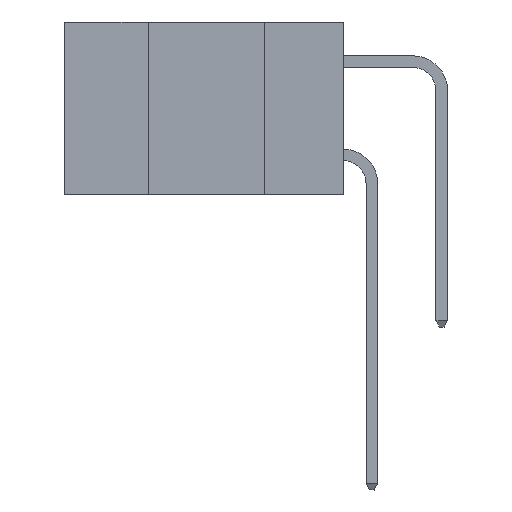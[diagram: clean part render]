
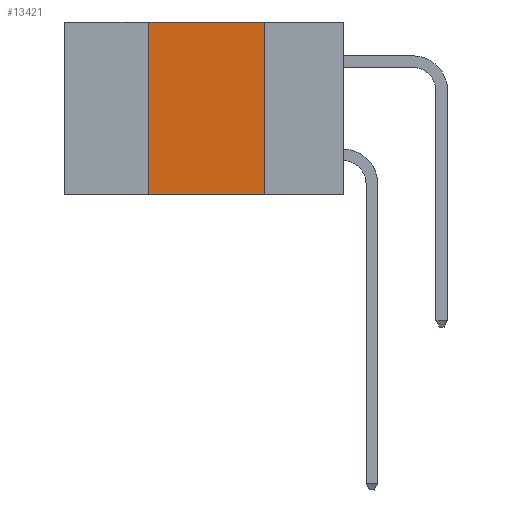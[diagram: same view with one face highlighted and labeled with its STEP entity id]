
A CAD part, left-side view. The second image highlights one B-rep face of the part: STEP entity #13421.
In plain terms, the highlighted planar face has unit normal (-1, 0, 0).
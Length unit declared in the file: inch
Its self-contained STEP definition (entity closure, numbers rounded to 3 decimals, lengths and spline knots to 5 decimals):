
#616 = ORIENTED_EDGE ( 'NONE', *, *, #10612, .F. ) ;
#756 = LINE ( 'NONE', #10088, #3636 ) ;
#978 = VECTOR ( 'NONE', #12851, 39.37008 ) ;
#1146 = CARTESIAN_POINT ( 'NONE',  ( 0., 0.6, -0.37 ) ) ;
#2519 = AXIS2_PLACEMENT_3D ( 'NONE', #10748, #4958, #7183 ) ;
#2936 = CARTESIAN_POINT ( 'NONE',  ( 0., 0.42, -0.37 ) ) ;
#2988 = VECTOR ( 'NONE', #4085, 39.37008 ) ;
#3181 = DIRECTION ( 'NONE',  ( 0., -1., 0. ) ) ;
#3538 = LINE ( 'NONE', #1146, #978 ) ;
#3636 = VECTOR ( 'NONE', #4363, 39.37008 ) ;
#3766 = VERTEX_POINT ( 'NONE', #12726 ) ;
#3930 = CARTESIAN_POINT ( 'NONE',  ( 0., 0.42, 0. ) ) ;
#4085 = DIRECTION ( 'NONE',  ( 0., 0., 1. ) ) ;
#4363 = DIRECTION ( 'NONE',  ( 0., 0., -1. ) ) ;
#4958 = DIRECTION ( 'NONE',  ( 1., 0., 0. ) ) ;
#5770 = CARTESIAN_POINT ( 'NONE',  ( 0., 0.17, -0.37 ) ) ;
#6140 = EDGE_LOOP ( 'NONE', ( #9791, #9254, #616, #9352 ) ) ;
#6281 = EDGE_CURVE ( 'NONE', #9557, #12571, #756, .T. ) ;
#7049 = VERTEX_POINT ( 'NONE', #3930 ) ;
#7183 = DIRECTION ( 'NONE',  ( 0., 0., -1. ) ) ;
#7984 = CARTESIAN_POINT ( 'NONE',  ( 0., 0.6, 0. ) ) ;
#8280 = EDGE_CURVE ( 'NONE', #3766, #12571, #3538, .T. ) ;
#8972 = EDGE_CURVE ( 'NONE', #7049, #9557, #10118, .T. ) ;
#9254 = ORIENTED_EDGE ( 'NONE', *, *, #8972, .F. ) ;
#9352 = ORIENTED_EDGE ( 'NONE', *, *, #8280, .T. ) ;
#9557 = VERTEX_POINT ( 'NONE', #10248 ) ;
#9791 = ORIENTED_EDGE ( 'NONE', *, *, #6281, .F. ) ;
#10088 = CARTESIAN_POINT ( 'NONE',  ( 0., 0.17, -0.37 ) ) ;
#10118 = LINE ( 'NONE', #7984, #12218 ) ;
#10248 = CARTESIAN_POINT ( 'NONE',  ( 0., 0.17, 0. ) ) ;
#10612 = EDGE_CURVE ( 'NONE', #3766, #7049, #14684, .T. ) ;
#10748 = CARTESIAN_POINT ( 'NONE',  ( 0., 0.6, 0. ) ) ;
#11752 = FACE_OUTER_BOUND ( 'NONE', #6140, .T. ) ;
#12218 = VECTOR ( 'NONE', #3181, 39.37008 ) ;
#12571 = VERTEX_POINT ( 'NONE', #5770 ) ;
#12726 = CARTESIAN_POINT ( 'NONE',  ( 0., 0.42, -0.37 ) ) ;
#12851 = DIRECTION ( 'NONE',  ( 0., -1., 0. ) ) ;
#13421 = ADVANCED_FACE ( 'NONE', ( #11752 ), #14199, .F. ) ;
#14199 = PLANE ( 'NONE',  #2519 ) ;
#14684 = LINE ( 'NONE', #2936, #2988 ) ;
